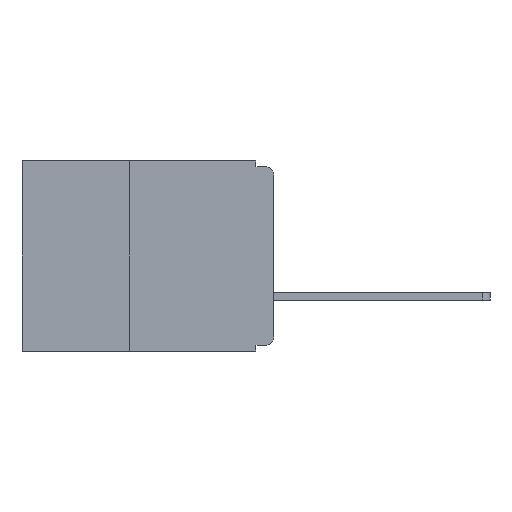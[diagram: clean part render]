
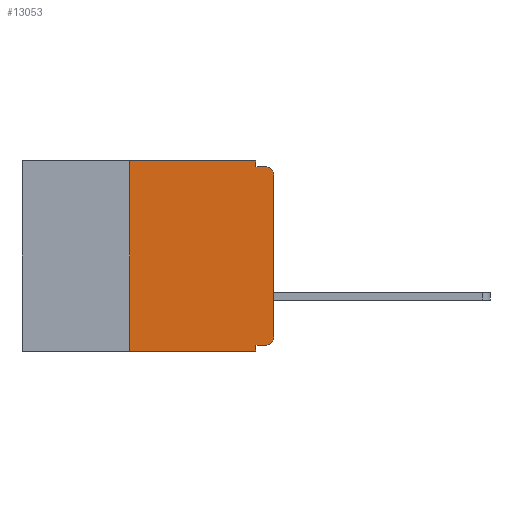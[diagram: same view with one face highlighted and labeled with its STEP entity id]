
A CAD part, left-side view. The second image highlights one B-rep face of the part: STEP entity #13053.
In plain terms, the highlighted planar face has unit normal (-1, 0, 0).
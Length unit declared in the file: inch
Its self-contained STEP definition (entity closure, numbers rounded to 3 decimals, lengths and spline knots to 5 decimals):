
#423 = ORIENTED_EDGE ( 'NONE', *, *, #17250, .T. ) ;
#445 = ORIENTED_EDGE ( 'NONE', *, *, #15036, .F. ) ;
#843 = VERTEX_POINT ( 'NONE', #1238 ) ;
#1014 = CARTESIAN_POINT ( 'NONE',  ( 0., 0.437, -0.33 ) ) ;
#1238 = CARTESIAN_POINT ( 'NONE',  ( 0., 0.25, -0.33 ) ) ;
#1309 = EDGE_CURVE ( 'NONE', #15673, #9459, #10983, .T. ) ;
#1506 = CARTESIAN_POINT ( 'NONE',  ( 0., 0.031, -0.32 ) ) ;
#1570 = EDGE_CURVE ( 'NONE', #19115, #13472, #15664, .T. ) ;
#1707 = VECTOR ( 'NONE', #5245, 39.37008 ) ;
#1761 = CARTESIAN_POINT ( 'NONE',  ( 0., 0., 0. ) ) ;
#2406 = CARTESIAN_POINT ( 'NONE',  ( 0., 0., -0.32 ) ) ;
#2779 = FACE_OUTER_BOUND ( 'NONE', #5772, .T. ) ;
#3281 = DIRECTION ( 'NONE',  ( 0., 0., -1. ) ) ;
#4508 = CARTESIAN_POINT ( 'NONE',  ( 0., 0., -0.01 ) ) ;
#4524 = VERTEX_POINT ( 'NONE', #9621 ) ;
#4980 = ORIENTED_EDGE ( 'NONE', *, *, #10298, .F. ) ;
#5128 = ORIENTED_EDGE ( 'NONE', *, *, #8485, .T. ) ;
#5245 = DIRECTION ( 'NONE',  ( 0., -1., 0. ) ) ;
#5610 = PLANE ( 'NONE',  #24117 ) ;
#5772 = EDGE_LOOP ( 'NONE', ( #6313, #5128, #4980, #19513, #11465, #12245, #423, #19610, #445, #9399 ) ) ;
#6313 = ORIENTED_EDGE ( 'NONE', *, *, #19584, .T. ) ;
#6440 = DIRECTION ( 'NONE',  ( 0., -1., 0. ) ) ;
#6483 = VECTOR ( 'NONE', #6440, 39.37008 ) ;
#6859 = CARTESIAN_POINT ( 'NONE',  ( 0., 0., -0.305 ) ) ;
#7520 = DIRECTION ( 'NONE',  ( 1., 0., 0. ) ) ;
#8008 = CIRCLE ( 'NONE', #15680, 0.015 ) ;
#8485 = EDGE_CURVE ( 'NONE', #10670, #12721, #8008, .T. ) ;
#9399 = ORIENTED_EDGE ( 'NONE', *, *, #1570, .T. ) ;
#9400 = LINE ( 'NONE', #1014, #23726 ) ;
#9435 = CARTESIAN_POINT ( 'NONE',  ( 0., 0., -0.025 ) ) ;
#9459 = VERTEX_POINT ( 'NONE', #14977 ) ;
#9621 = CARTESIAN_POINT ( 'NONE',  ( 0., 0.031, -0.01 ) ) ;
#9735 = LINE ( 'NONE', #17880, #10893 ) ;
#10096 = DIRECTION ( 'NONE',  ( -1., 0., 0. ) ) ;
#10298 = EDGE_CURVE ( 'NONE', #4524, #12721, #21472, .T. ) ;
#10629 = DIRECTION ( 'NONE',  ( 0., 0., -1. ) ) ;
#10670 = VERTEX_POINT ( 'NONE', #9435 ) ;
#10893 = VECTOR ( 'NONE', #12227, 39.37008 ) ;
#10983 = LINE ( 'NONE', #11643, #20340 ) ;
#11066 = LINE ( 'NONE', #1761, #14883 ) ;
#11197 = DIRECTION ( 'NONE',  ( 0., 0., 1. ) ) ;
#11465 = ORIENTED_EDGE ( 'NONE', *, *, #16753, .F. ) ;
#11643 = CARTESIAN_POINT ( 'NONE',  ( 0., 0.031, -0.33 ) ) ;
#12227 = DIRECTION ( 'NONE',  ( 0., 0., -1. ) ) ;
#12245 = ORIENTED_EDGE ( 'NONE', *, *, #16285, .F. ) ;
#12721 = VERTEX_POINT ( 'NONE', #17873 ) ;
#12960 = VERTEX_POINT ( 'NONE', #14717 ) ;
#13053 = ADVANCED_FACE ( 'NONE', ( #2779 ), #5610, .F. ) ;
#13472 = VERTEX_POINT ( 'NONE', #6859 ) ;
#13532 = DIRECTION ( 'NONE',  ( -1., 0., 0. ) ) ;
#13694 = CARTESIAN_POINT ( 'NONE',  ( 0., 0.015, -0.305 ) ) ;
#14717 = CARTESIAN_POINT ( 'NONE',  ( 0., 0.25, 0. ) ) ;
#14883 = VECTOR ( 'NONE', #11197, 39.37008 ) ;
#14977 = CARTESIAN_POINT ( 'NONE',  ( 0., 0.031, -0.33 ) ) ;
#15036 = EDGE_CURVE ( 'NONE', #19115, #15673, #19500, .T. ) ;
#15043 = CARTESIAN_POINT ( 'NONE',  ( 0., 0.437, 0. ) ) ;
#15515 = DIRECTION ( 'NONE',  ( 0., 1., 0. ) ) ;
#15581 = AXIS2_PLACEMENT_3D ( 'NONE', #13694, #13532, #10629 ) ;
#15587 = LINE ( 'NONE', #16564, #1707 ) ;
#15664 = CIRCLE ( 'NONE', #15581, 0.015 ) ;
#15673 = VERTEX_POINT ( 'NONE', #1506 ) ;
#15680 = AXIS2_PLACEMENT_3D ( 'NONE', #21295, #10096, #23165 ) ;
#15971 = CARTESIAN_POINT ( 'NONE',  ( 0., 0.031, 0. ) ) ;
#16042 = DIRECTION ( 'NONE',  ( 0., -1., 0. ) ) ;
#16285 = EDGE_CURVE ( 'NONE', #843, #12960, #23482, .T. ) ;
#16564 = CARTESIAN_POINT ( 'NONE',  ( 0., 0.437, 0. ) ) ;
#16579 = EDGE_CURVE ( 'NONE', #21072, #4524, #9735, .T. ) ;
#16753 = EDGE_CURVE ( 'NONE', #12960, #21072, #15587, .T. ) ;
#16793 = VECTOR ( 'NONE', #18881, 39.37008 ) ;
#17250 = EDGE_CURVE ( 'NONE', #843, #9459, #9400, .T. ) ;
#17873 = CARTESIAN_POINT ( 'NONE',  ( 0., 0.015, -0.01 ) ) ;
#17880 = CARTESIAN_POINT ( 'NONE',  ( 0., 0.031, 0. ) ) ;
#18881 = DIRECTION ( 'NONE',  ( 0., 0., 1. ) ) ;
#18903 = VECTOR ( 'NONE', #15515, 39.37008 ) ;
#19115 = VERTEX_POINT ( 'NONE', #19189 ) ;
#19189 = CARTESIAN_POINT ( 'NONE',  ( 0., 0.015, -0.32 ) ) ;
#19500 = LINE ( 'NONE', #2406, #18903 ) ;
#19513 = ORIENTED_EDGE ( 'NONE', *, *, #16579, .F. ) ;
#19584 = EDGE_CURVE ( 'NONE', #13472, #10670, #11066, .T. ) ;
#19610 = ORIENTED_EDGE ( 'NONE', *, *, #1309, .F. ) ;
#20340 = VECTOR ( 'NONE', #3281, 39.37008 ) ;
#20664 = DIRECTION ( 'NONE',  ( 0., 0., -1. ) ) ;
#20731 = CARTESIAN_POINT ( 'NONE',  ( 0., 0.25, -0.33 ) ) ;
#21072 = VERTEX_POINT ( 'NONE', #15971 ) ;
#21295 = CARTESIAN_POINT ( 'NONE',  ( 0., 0.015, -0.025 ) ) ;
#21472 = LINE ( 'NONE', #4508, #6483 ) ;
#23165 = DIRECTION ( 'NONE',  ( 0., 0., -1. ) ) ;
#23482 = LINE ( 'NONE', #20731, #16793 ) ;
#23726 = VECTOR ( 'NONE', #16042, 39.37008 ) ;
#24117 = AXIS2_PLACEMENT_3D ( 'NONE', #15043, #7520, #20664 ) ;
